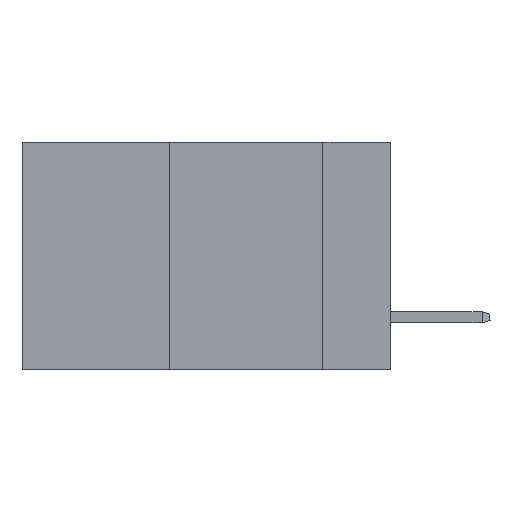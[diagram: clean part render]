
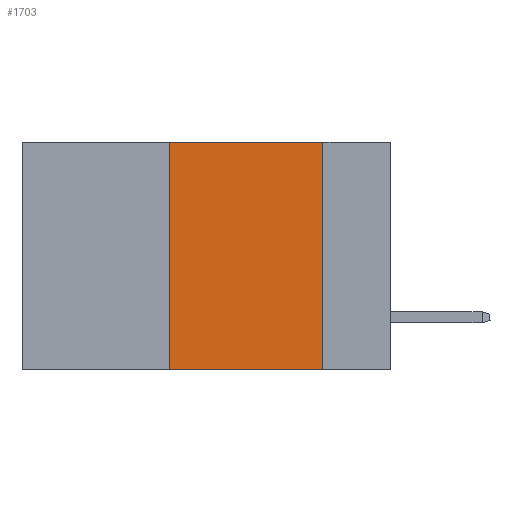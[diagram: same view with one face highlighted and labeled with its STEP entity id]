
A CAD part, left-side view. The second image highlights one B-rep face of the part: STEP entity #1703.
In plain terms, the highlighted planar face has unit normal (-1, 0, 0).
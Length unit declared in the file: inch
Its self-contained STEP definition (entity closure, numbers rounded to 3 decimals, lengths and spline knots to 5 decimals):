
#281 = CARTESIAN_POINT ( 'NONE',  ( 0., 0.6, -0.37 ) ) ;
#1703 = ADVANCED_FACE ( 'NONE', ( #17634 ), #20362, .F. ) ;
#2585 = DIRECTION ( 'NONE',  ( 0., -1., 0. ) ) ;
#2897 = LINE ( 'NONE', #28392, #24881 ) ;
#2912 = VECTOR ( 'NONE', #2585, 39.37008 ) ;
#3627 = ORIENTED_EDGE ( 'NONE', *, *, #29099, .F. ) ;
#3663 = VECTOR ( 'NONE', #13354, 39.37008 ) ;
#3815 = DIRECTION ( 'NONE',  ( 0., -1., 0. ) ) ;
#5714 = DIRECTION ( 'NONE',  ( 0., 0., 1. ) ) ;
#6293 = CARTESIAN_POINT ( 'NONE',  ( 0., 0.36, -0.37 ) ) ;
#6889 = AXIS2_PLACEMENT_3D ( 'NONE', #24675, #17800, #22641 ) ;
#9896 = ORIENTED_EDGE ( 'NONE', *, *, #16167, .F. ) ;
#11398 = VERTEX_POINT ( 'NONE', #6293 ) ;
#11423 = LINE ( 'NONE', #281, #2912 ) ;
#12802 = VERTEX_POINT ( 'NONE', #27792 ) ;
#13354 = DIRECTION ( 'NONE',  ( 0., 0., -1. ) ) ;
#14777 = VERTEX_POINT ( 'NONE', #14848 ) ;
#14848 = CARTESIAN_POINT ( 'NONE',  ( 0., 0.36, 0. ) ) ;
#16167 = EDGE_CURVE ( 'NONE', #12802, #19117, #25982, .T. ) ;
#17268 = EDGE_CURVE ( 'NONE', #14777, #12802, #27695, .T. ) ;
#17634 = FACE_OUTER_BOUND ( 'NONE', #24294, .T. ) ;
#17800 = DIRECTION ( 'NONE',  ( 1., 0., 0. ) ) ;
#19117 = VERTEX_POINT ( 'NONE', #25065 ) ;
#19494 = CARTESIAN_POINT ( 'NONE',  ( 0., 0.11, 0. ) ) ;
#20362 = PLANE ( 'NONE',  #6889 ) ;
#21673 = VECTOR ( 'NONE', #3815, 39.37008 ) ;
#22641 = DIRECTION ( 'NONE',  ( 0., 0., -1. ) ) ;
#23808 = CARTESIAN_POINT ( 'NONE',  ( 0., 0.6, 0. ) ) ;
#24294 = EDGE_LOOP ( 'NONE', ( #9896, #27528, #3627, #25901 ) ) ;
#24675 = CARTESIAN_POINT ( 'NONE',  ( 0., 0.6, 0. ) ) ;
#24881 = VECTOR ( 'NONE', #5714, 39.37008 ) ;
#25065 = CARTESIAN_POINT ( 'NONE',  ( 0., 0.11, -0.37 ) ) ;
#25901 = ORIENTED_EDGE ( 'NONE', *, *, #28113, .T. ) ;
#25982 = LINE ( 'NONE', #19494, #3663 ) ;
#27528 = ORIENTED_EDGE ( 'NONE', *, *, #17268, .F. ) ;
#27695 = LINE ( 'NONE', #23808, #21673 ) ;
#27792 = CARTESIAN_POINT ( 'NONE',  ( 0., 0.11, 0. ) ) ;
#28113 = EDGE_CURVE ( 'NONE', #11398, #19117, #11423, .T. ) ;
#28392 = CARTESIAN_POINT ( 'NONE',  ( 0., 0.36, 0. ) ) ;
#29099 = EDGE_CURVE ( 'NONE', #11398, #14777, #2897, .T. ) ;
